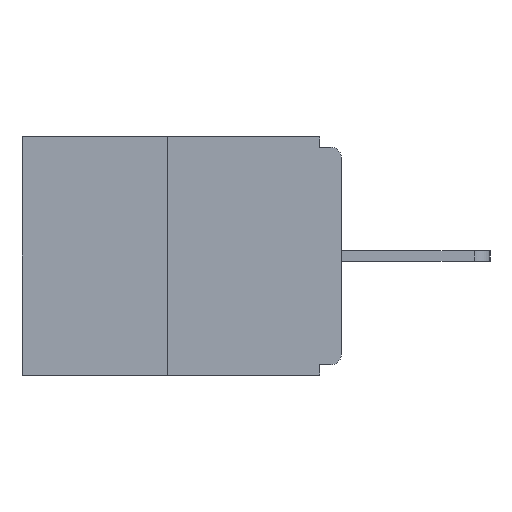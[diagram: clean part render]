
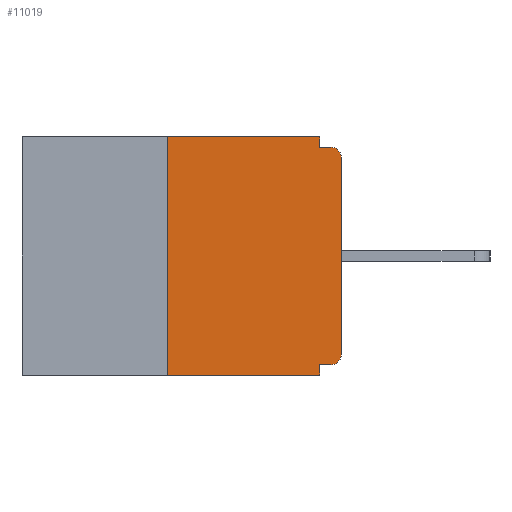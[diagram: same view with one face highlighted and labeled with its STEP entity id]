
A CAD part, left-side view. The second image highlights one B-rep face of the part: STEP entity #11019.
In plain terms, the highlighted planar face has unit normal (-1, 0, 0).
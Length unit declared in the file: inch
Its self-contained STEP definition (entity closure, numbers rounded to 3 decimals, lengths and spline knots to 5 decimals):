
#182 = LINE ( 'NONE', #11404, #4313 ) ;
#243 = CARTESIAN_POINT ( 'NONE',  ( 0., 0.015, -0.313 ) ) ;
#304 = CARTESIAN_POINT ( 'NONE',  ( 0., 0.015, -0.03 ) ) ;
#418 = VERTEX_POINT ( 'NONE', #10257 ) ;
#456 = CARTESIAN_POINT ( 'NONE',  ( 0., 0., -0.313 ) ) ;
#506 = VECTOR ( 'NONE', #8946, 39.37008 ) ;
#550 = LINE ( 'NONE', #3381, #9041 ) ;
#701 = DIRECTION ( 'NONE',  ( 1., 0., 0. ) ) ;
#1120 = DIRECTION ( 'NONE',  ( 0., 0., 1. ) ) ;
#1333 = EDGE_LOOP ( 'NONE', ( #4705, #6630, #1625, #3435, #10051, #5268, #11299, #8402, #9217, #4595 ) ) ;
#1439 = VERTEX_POINT ( 'NONE', #12227 ) ;
#1625 = ORIENTED_EDGE ( 'NONE', *, *, #5100, .T. ) ;
#1827 = EDGE_CURVE ( 'NONE', #1439, #2746, #7465, .T. ) ;
#2195 = CARTESIAN_POINT ( 'NONE',  ( 0., 0.031, -0.015 ) ) ;
#2220 = DIRECTION ( 'NONE',  ( 0., 0., -1. ) ) ;
#2265 = LINE ( 'NONE', #10899, #4863 ) ;
#2285 = CIRCLE ( 'NONE', #3679, 0.015 ) ;
#2355 = VECTOR ( 'NONE', #11973, 39.37008 ) ;
#2394 = DIRECTION ( 'NONE',  ( 0., 0., 1. ) ) ;
#2443 = CARTESIAN_POINT ( 'NONE',  ( 0., 0.25, 0. ) ) ;
#2536 = DIRECTION ( 'NONE',  ( 0., 0., -1. ) ) ;
#2562 = CARTESIAN_POINT ( 'NONE',  ( 0., 0.031, 0. ) ) ;
#2638 = VERTEX_POINT ( 'NONE', #8848 ) ;
#2746 = VERTEX_POINT ( 'NONE', #7437 ) ;
#2968 = CARTESIAN_POINT ( 'NONE',  ( 0., 0., 0. ) ) ;
#3203 = EDGE_CURVE ( 'NONE', #7071, #1439, #4591, .T. ) ;
#3291 = FACE_OUTER_BOUND ( 'NONE', #1333, .T. ) ;
#3381 = CARTESIAN_POINT ( 'NONE',  ( 0., 0.031, 0. ) ) ;
#3435 = ORIENTED_EDGE ( 'NONE', *, *, #1827, .F. ) ;
#3475 = AXIS2_PLACEMENT_3D ( 'NONE', #243, #7625, #10600 ) ;
#3679 = AXIS2_PLACEMENT_3D ( 'NONE', #304, #8049, #10954 ) ;
#3754 = EDGE_CURVE ( 'NONE', #7071, #9819, #5082, .T. ) ;
#3872 = VERTEX_POINT ( 'NONE', #10783 ) ;
#4130 = CARTESIAN_POINT ( 'NONE',  ( 0., 0.46, -0.343 ) ) ;
#4313 = VECTOR ( 'NONE', #7818, 39.37008 ) ;
#4591 = LINE ( 'NONE', #10302, #2355 ) ;
#4595 = ORIENTED_EDGE ( 'NONE', *, *, #8015, .F. ) ;
#4705 = ORIENTED_EDGE ( 'NONE', *, *, #7165, .F. ) ;
#4863 = VECTOR ( 'NONE', #2394, 39.37008 ) ;
#4929 = VECTOR ( 'NONE', #2536, 39.37008 ) ;
#5037 = EDGE_CURVE ( 'NONE', #2638, #6625, #2265, .T. ) ;
#5082 = CIRCLE ( 'NONE', #3475, 0.015 ) ;
#5100 = EDGE_CURVE ( 'NONE', #2638, #2746, #6204, .T. ) ;
#5185 = CARTESIAN_POINT ( 'NONE',  ( 0., 0.46, 0. ) ) ;
#5245 = PLANE ( 'NONE',  #5556 ) ;
#5268 = ORIENTED_EDGE ( 'NONE', *, *, #3754, .T. ) ;
#5556 = AXIS2_PLACEMENT_3D ( 'NONE', #11798, #701, #9879 ) ;
#6204 = LINE ( 'NONE', #4130, #10428 ) ;
#6625 = VERTEX_POINT ( 'NONE', #2443 ) ;
#6630 = ORIENTED_EDGE ( 'NONE', *, *, #5037, .F. ) ;
#6689 = VERTEX_POINT ( 'NONE', #2562 ) ;
#7071 = VERTEX_POINT ( 'NONE', #9811 ) ;
#7165 = EDGE_CURVE ( 'NONE', #6625, #6689, #10811, .T. ) ;
#7437 = CARTESIAN_POINT ( 'NONE',  ( 0., 0.031, -0.343 ) ) ;
#7465 = LINE ( 'NONE', #12212, #4929 ) ;
#7625 = DIRECTION ( 'NONE',  ( -1., 0., 0. ) ) ;
#7818 = DIRECTION ( 'NONE',  ( 0., -1., 0. ) ) ;
#7925 = EDGE_CURVE ( 'NONE', #3872, #418, #2285, .T. ) ;
#8015 = EDGE_CURVE ( 'NONE', #6689, #8179, #550, .T. ) ;
#8049 = DIRECTION ( 'NONE',  ( -1., 0., 0. ) ) ;
#8179 = VERTEX_POINT ( 'NONE', #2195 ) ;
#8402 = ORIENTED_EDGE ( 'NONE', *, *, #7925, .T. ) ;
#8848 = CARTESIAN_POINT ( 'NONE',  ( 0., 0.25, -0.343 ) ) ;
#8946 = DIRECTION ( 'NONE',  ( 0., -1., 0. ) ) ;
#9041 = VECTOR ( 'NONE', #2220, 39.37008 ) ;
#9217 = ORIENTED_EDGE ( 'NONE', *, *, #10440, .F. ) ;
#9542 = LINE ( 'NONE', #2968, #9611 ) ;
#9611 = VECTOR ( 'NONE', #1120, 39.37008 ) ;
#9811 = CARTESIAN_POINT ( 'NONE',  ( 0., 0.015, -0.328 ) ) ;
#9819 = VERTEX_POINT ( 'NONE', #456 ) ;
#9879 = DIRECTION ( 'NONE',  ( 0., 0., -1. ) ) ;
#9972 = DIRECTION ( 'NONE',  ( 0., -1., 0. ) ) ;
#10051 = ORIENTED_EDGE ( 'NONE', *, *, #3203, .F. ) ;
#10257 = CARTESIAN_POINT ( 'NONE',  ( 0., 0.015, -0.015 ) ) ;
#10302 = CARTESIAN_POINT ( 'NONE',  ( 0., 0., -0.328 ) ) ;
#10428 = VECTOR ( 'NONE', #9972, 39.37008 ) ;
#10440 = EDGE_CURVE ( 'NONE', #8179, #418, #182, .T. ) ;
#10600 = DIRECTION ( 'NONE',  ( 0., 0., -1. ) ) ;
#10783 = CARTESIAN_POINT ( 'NONE',  ( 0., 0., -0.03 ) ) ;
#10811 = LINE ( 'NONE', #5185, #506 ) ;
#10899 = CARTESIAN_POINT ( 'NONE',  ( 0., 0.25, 0. ) ) ;
#10954 = DIRECTION ( 'NONE',  ( 0., 0., -1. ) ) ;
#11019 = ADVANCED_FACE ( 'NONE', ( #3291 ), #5245, .F. ) ;
#11299 = ORIENTED_EDGE ( 'NONE', *, *, #11722, .T. ) ;
#11404 = CARTESIAN_POINT ( 'NONE',  ( 0., 0., -0.015 ) ) ;
#11722 = EDGE_CURVE ( 'NONE', #9819, #3872, #9542, .T. ) ;
#11798 = CARTESIAN_POINT ( 'NONE',  ( 0., 0.46, 0. ) ) ;
#11973 = DIRECTION ( 'NONE',  ( 0., 1., 0. ) ) ;
#12212 = CARTESIAN_POINT ( 'NONE',  ( 0., 0.031, -0.343 ) ) ;
#12227 = CARTESIAN_POINT ( 'NONE',  ( 0., 0.031, -0.328 ) ) ;
